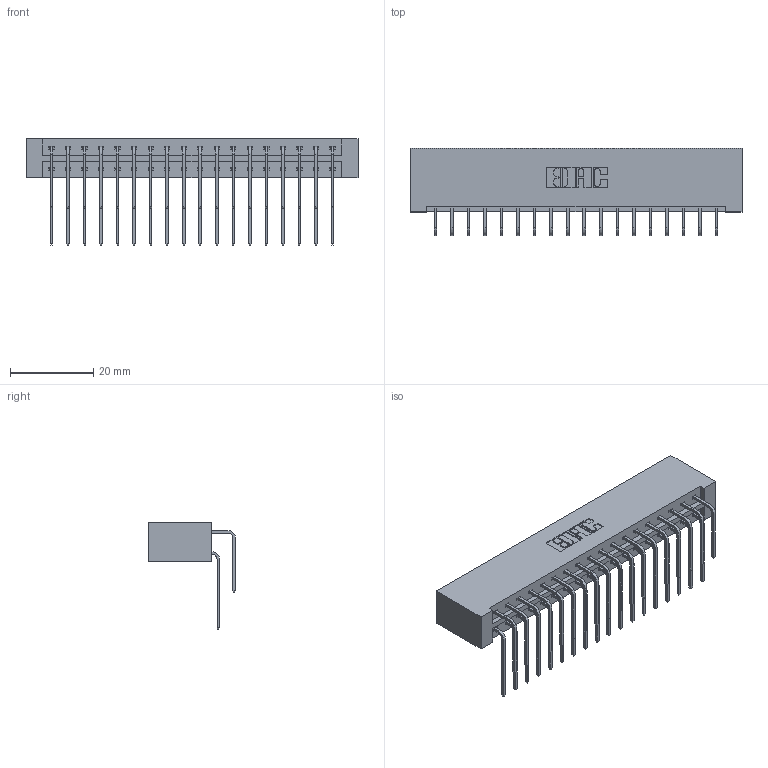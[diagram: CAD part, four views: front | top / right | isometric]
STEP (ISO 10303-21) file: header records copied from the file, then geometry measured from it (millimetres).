
FILE_DESCRIPTION (( 'STEP AP203' ), '1' );
FILE_NAME ('833-036-559-201.STEP', '2020-06-03T04:07:51', ( '' ), ( '' ), 'SwSTEP 2.0', 'SolidWorks 2020', '' );
FILE_SCHEMA (( 'CONFIG_CONTROL_DESIGN' ));
Length unit declared in the file: inch
Products named in the file (4): 833 Part_Lugless; 833-036-559-201; 345-292-001_559 Tail - 2; 345-292-001_558 559 Tail - 1
Assembly tree (37 placements, depth 2):
  833-036-559-201
    833 Part_Lugless
    345-292-001_558 559 Tail - 1  x18
    345-292-001_559 Tail - 2  x18
Bounding box: 79.58 x 20.9 x 25.53 mm (x, y, z)
Volume: 8739.9 mm3; surface area: 11133.7 mm2
Topology: 37 solids, 37 shells, 2050 faces, 6083 edges, 4006 vertices
Faces by surface type: plane 1434, cylinder 616
Entity records: 16191 total; most frequent: CARTESIAN_POINT 2761, ORIENTED_EDGE 2646, DIRECTION 2375, EDGE_CURVE 1323, LINE 1163, VECTOR 1163, VERTEX_POINT 878, AXIS2_PLACEMENT_3D 606
